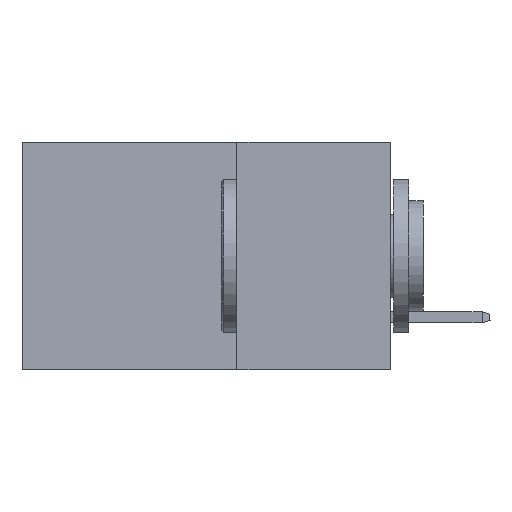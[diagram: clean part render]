
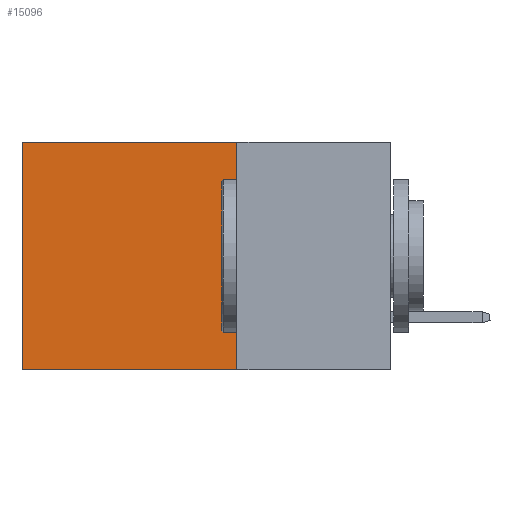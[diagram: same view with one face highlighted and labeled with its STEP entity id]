
A CAD part, left-side view. The second image highlights one B-rep face of the part: STEP entity #15096.
In plain terms, the highlighted planar face has unit normal (-1, 0, 0).
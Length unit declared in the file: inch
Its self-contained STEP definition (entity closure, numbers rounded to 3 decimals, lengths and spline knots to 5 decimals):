
#450 = LINE ( 'NONE', #48807, #49559 ) ;
#2387 = DIRECTION ( 'NONE',  ( 0., 1., 0. ) ) ;
#3249 = EDGE_CURVE ( 'NONE', #4607, #16076, #37524, .T. ) ;
#4607 = VERTEX_POINT ( 'NONE', #6631 ) ;
#4997 = ORIENTED_EDGE ( 'NONE', *, *, #49357, .T. ) ;
#5441 = ORIENTED_EDGE ( 'NONE', *, *, #26217, .T. ) ;
#6029 = CARTESIAN_POINT ( 'NONE',  ( 0.2875, 0.25, 0. ) ) ;
#6614 = ORIENTED_EDGE ( 'NONE', *, *, #3249, .F. ) ;
#6631 = CARTESIAN_POINT ( 'NONE',  ( 0.2875, 0.25, -0.37 ) ) ;
#7229 = CARTESIAN_POINT ( 'NONE',  ( 0.2875, 0.25, 0. ) ) ;
#8218 = DIRECTION ( 'NONE',  ( 0., 1., 0. ) ) ;
#8251 = EDGE_CURVE ( 'NONE', #28221, #4607, #10221, .T. ) ;
#9788 = DIRECTION ( 'NONE',  ( 0., 0., -1. ) ) ;
#10221 = LINE ( 'NONE', #36842, #38157 ) ;
#11623 = CARTESIAN_POINT ( 'NONE',  ( 0.2875, 0.6, -0.37 ) ) ;
#12593 = VECTOR ( 'NONE', #2387, 39.37008 ) ;
#15096 = ADVANCED_FACE ( 'NONE', ( #26963 ), #44440, .F. ) ;
#16076 = VERTEX_POINT ( 'NONE', #11623 ) ;
#18667 = EDGE_LOOP ( 'NONE', ( #5441, #6614, #24161, #4997 ) ) ;
#20716 = DIRECTION ( 'NONE',  ( 0., 0., -1. ) ) ;
#24161 = ORIENTED_EDGE ( 'NONE', *, *, #8251, .F. ) ;
#24509 = VERTEX_POINT ( 'NONE', #34834 ) ;
#24760 = DIRECTION ( 'NONE',  ( 0., 0., -1. ) ) ;
#26217 = EDGE_CURVE ( 'NONE', #24509, #16076, #450, .T. ) ;
#26963 = FACE_OUTER_BOUND ( 'NONE', #18667, .T. ) ;
#28221 = VERTEX_POINT ( 'NONE', #6029 ) ;
#28803 = DIRECTION ( 'NONE',  ( 1., 0., 0. ) ) ;
#34834 = CARTESIAN_POINT ( 'NONE',  ( 0.2875, 0.6, 0. ) ) ;
#34943 = VECTOR ( 'NONE', #8218, 39.37008 ) ;
#36614 = AXIS2_PLACEMENT_3D ( 'NONE', #43941, #28803, #24760 ) ;
#36842 = CARTESIAN_POINT ( 'NONE',  ( 0.2875, 0.25, 0. ) ) ;
#37524 = LINE ( 'NONE', #48669, #12593 ) ;
#38157 = VECTOR ( 'NONE', #20716, 39.37008 ) ;
#42242 = LINE ( 'NONE', #7229, #34943 ) ;
#43941 = CARTESIAN_POINT ( 'NONE',  ( 0.2875, 0.25, 0. ) ) ;
#44440 = PLANE ( 'NONE',  #36614 ) ;
#48669 = CARTESIAN_POINT ( 'NONE',  ( 0.2875, 0.25, -0.37 ) ) ;
#48807 = CARTESIAN_POINT ( 'NONE',  ( 0.2875, 0.6, 0. ) ) ;
#49357 = EDGE_CURVE ( 'NONE', #28221, #24509, #42242, .T. ) ;
#49559 = VECTOR ( 'NONE', #9788, 39.37008 ) ;
